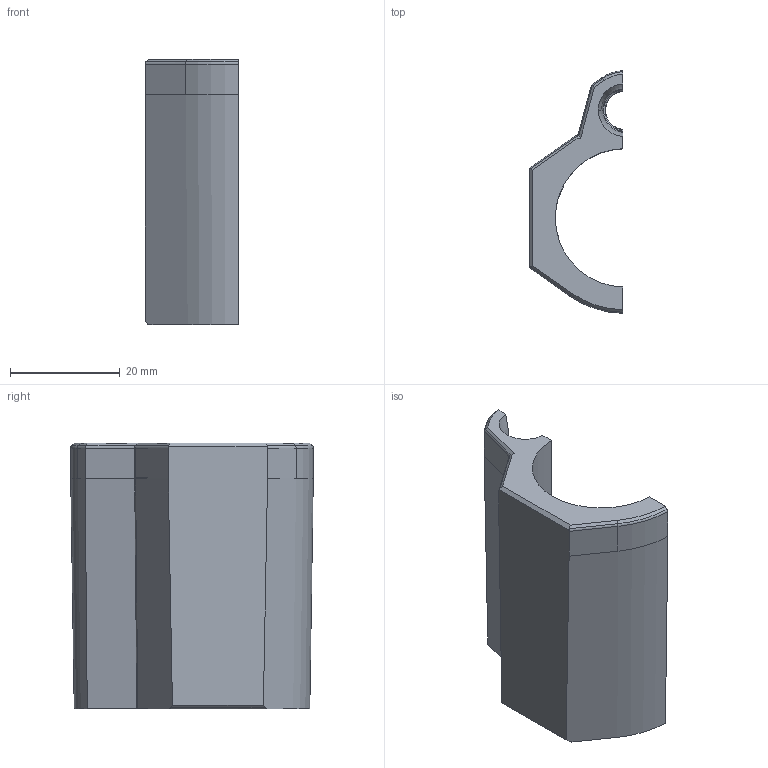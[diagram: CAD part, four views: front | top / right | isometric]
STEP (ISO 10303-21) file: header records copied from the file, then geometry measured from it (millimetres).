
FILE_DESCRIPTION (( 'STEP AP203' ), '1' );
FILE_NAME ('Orca Barrel Mount Right V5.3.STEP', '2023-01-20T23:41:40', ( '' ), ( '' ), 'SwSTEP 2.0', 'SolidWorks 2021', '' );
FILE_SCHEMA (( 'CONFIG_CONTROL_DESIGN' ));
Length unit declared in the file: inch
Products named in the file (1): Orca Barrel Mount Right V5.3
Bounding box: 17.09 x 44.11 x 48.34 mm (x, y, z)
Volume: 12349.8 mm3; surface area: 6779.6 mm2
Topology: 1 solids, 1 shells, 132 faces, 357 edges, 231 vertices
Faces by surface type: bspline 58, cylinder 25, plane 24, torus 20, cone 5
Entity records: 11784 total; most frequent: CARTESIAN_POINT 8938, ORIENTED_EDGE 714, DIRECTION 358, EDGE_CURVE 357, VERTEX_POINT 231, B_SPLINE_CURVE_WITH_KNOTS 200, AXIS2_PLACEMENT_3D 136, EDGE_LOOP 136
